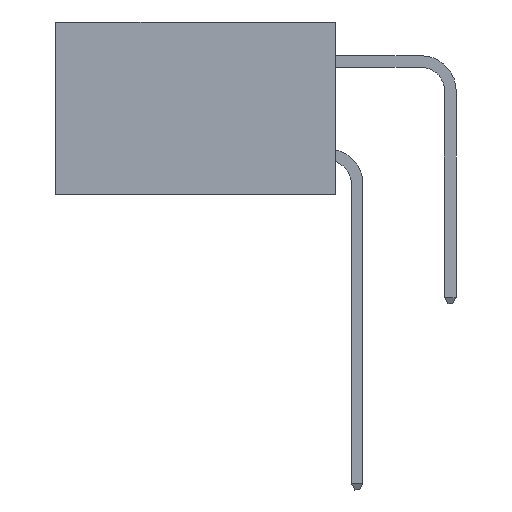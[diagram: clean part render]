
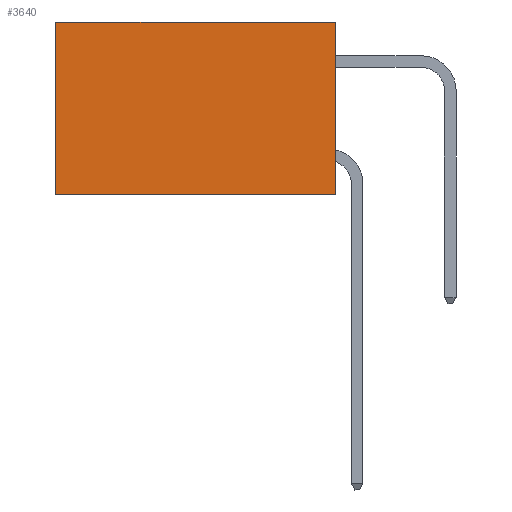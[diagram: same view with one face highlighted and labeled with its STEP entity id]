
A CAD part, left-side view. The second image highlights one B-rep face of the part: STEP entity #3640.
In plain terms, the highlighted planar face has unit normal (-1, 0, 0).
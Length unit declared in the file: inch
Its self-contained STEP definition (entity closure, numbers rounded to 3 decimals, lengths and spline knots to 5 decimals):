
#240 = CARTESIAN_POINT ( 'NONE',  ( 0.2875, 0., -0.37 ) ) ;
#410 = AXIS2_PLACEMENT_3D ( 'NONE', #2982, #7458, #3644 ) ;
#463 = VECTOR ( 'NONE', #36022, 39.37008 ) ;
#776 = EDGE_LOOP ( 'NONE', ( #27873, #32276, #33211, #3971 ) ) ;
#954 = CARTESIAN_POINT ( 'NONE',  ( 0.2875, 0., 0. ) ) ;
#2982 = CARTESIAN_POINT ( 'NONE',  ( 0.2875, 0., 0. ) ) ;
#3305 = CARTESIAN_POINT ( 'NONE',  ( 0.2875, 0.6, 0. ) ) ;
#3640 = ADVANCED_FACE ( 'NONE', ( #20704 ), #29626, .F. ) ;
#3644 = DIRECTION ( 'NONE',  ( 0., 0., -1. ) ) ;
#3790 = LINE ( 'NONE', #240, #463 ) ;
#3971 = ORIENTED_EDGE ( 'NONE', *, *, #13637, .T. ) ;
#4441 = CARTESIAN_POINT ( 'NONE',  ( 0.2875, 0.6, 0. ) ) ;
#4795 = EDGE_CURVE ( 'NONE', #26668, #32546, #8876, .T. ) ;
#7169 = DIRECTION ( 'NONE',  ( 0., 0., -1. ) ) ;
#7452 = EDGE_CURVE ( 'NONE', #22425, #32546, #3790, .T. ) ;
#7458 = DIRECTION ( 'NONE',  ( 1., 0., 0. ) ) ;
#8876 = LINE ( 'NONE', #4441, #20103 ) ;
#12081 = DIRECTION ( 'NONE',  ( 0., 1., 0. ) ) ;
#13637 = EDGE_CURVE ( 'NONE', #32264, #26668, #22817, .T. ) ;
#17933 = CARTESIAN_POINT ( 'NONE',  ( 0.2875, 0., -0.37 ) ) ;
#17995 = CARTESIAN_POINT ( 'NONE',  ( 0.2875, 0., 0. ) ) ;
#20103 = VECTOR ( 'NONE', #22560, 39.37008 ) ;
#20704 = FACE_OUTER_BOUND ( 'NONE', #776, .T. ) ;
#22425 = VERTEX_POINT ( 'NONE', #17933 ) ;
#22560 = DIRECTION ( 'NONE',  ( 0., 0., -1. ) ) ;
#22817 = LINE ( 'NONE', #17995, #30768 ) ;
#26668 = VERTEX_POINT ( 'NONE', #3305 ) ;
#26774 = VECTOR ( 'NONE', #7169, 39.37008 ) ;
#27873 = ORIENTED_EDGE ( 'NONE', *, *, #4795, .T. ) ;
#29073 = EDGE_CURVE ( 'NONE', #32264, #22425, #29128, .T. ) ;
#29128 = LINE ( 'NONE', #954, #26774 ) ;
#29626 = PLANE ( 'NONE',  #410 ) ;
#30768 = VECTOR ( 'NONE', #12081, 39.37008 ) ;
#31515 = CARTESIAN_POINT ( 'NONE',  ( 0.2875, 0., 0. ) ) ;
#32264 = VERTEX_POINT ( 'NONE', #31515 ) ;
#32276 = ORIENTED_EDGE ( 'NONE', *, *, #7452, .F. ) ;
#32546 = VERTEX_POINT ( 'NONE', #35977 ) ;
#33211 = ORIENTED_EDGE ( 'NONE', *, *, #29073, .F. ) ;
#35977 = CARTESIAN_POINT ( 'NONE',  ( 0.2875, 0.6, -0.37 ) ) ;
#36022 = DIRECTION ( 'NONE',  ( 0., 1., 0. ) ) ;
